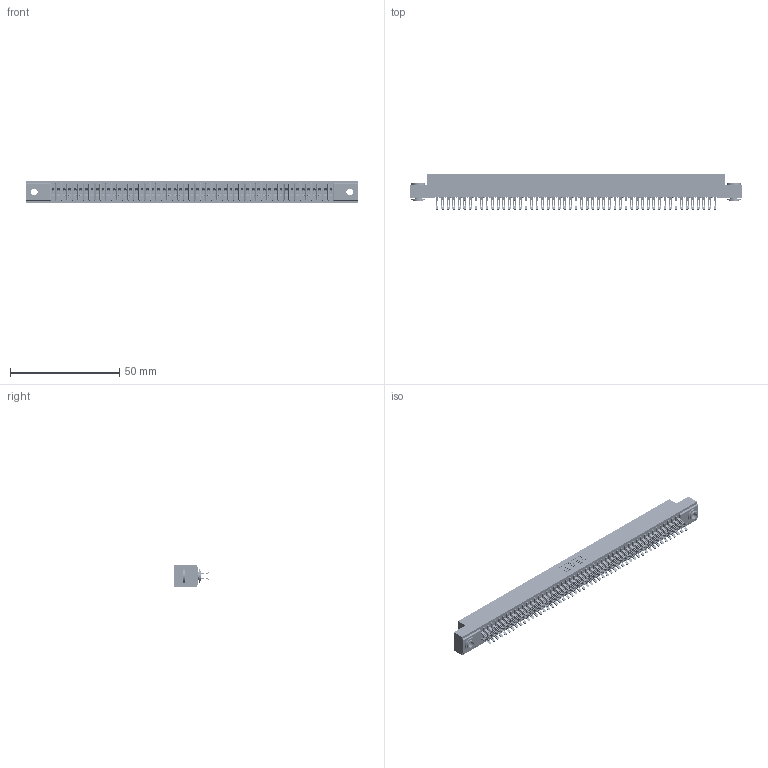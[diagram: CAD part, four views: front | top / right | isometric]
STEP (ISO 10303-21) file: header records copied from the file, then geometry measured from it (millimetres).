
FILE_DESCRIPTION (( 'STEP AP203' ), '1' );
FILE_NAME ('341-102-555-203.STEP', '2018-08-08T11:15:57', ( '' ), ( '' ), 'SwSTEP 2.0', 'SolidWorks 2016', '' );
FILE_SCHEMA (( 'CONFIG_CONTROL_DESIGN' ));
Length unit declared in the file: inch
Products named in the file (4): 341-292-001_341-292-155; 345-250-002_345-250-002-102; 341-102-555-203; 341 Part_.156 (3.96) Dia Mounting Holes
Assembly tree (105 placements, depth 2):
  341-102-555-203
    341 Part_.156 (3.96) Dia Mounting Holes
    341-292-001_341-292-155  x102
    345-250-002_345-250-002-102  x2
Bounding box: 151.76 x 16.31 x 10.16 mm (x, y, z)
Volume: 11346 mm3; surface area: 21501.4 mm2
Topology: 105 solids, 105 shells, 8124 faces, 24245 edges, 15782 vertices
Faces by surface type: plane 4376, cylinder 3536, sphere 104, torus 100, cone 8
Entity records: 62057 total; most frequent: CARTESIAN_POINT 10312, ORIENTED_EDGE 10230, DIRECTION 10007, EDGE_CURVE 5115, LINE 4117, VECTOR 4117, VERTEX_POINT 3234, AXIS2_PLACEMENT_3D 2945
